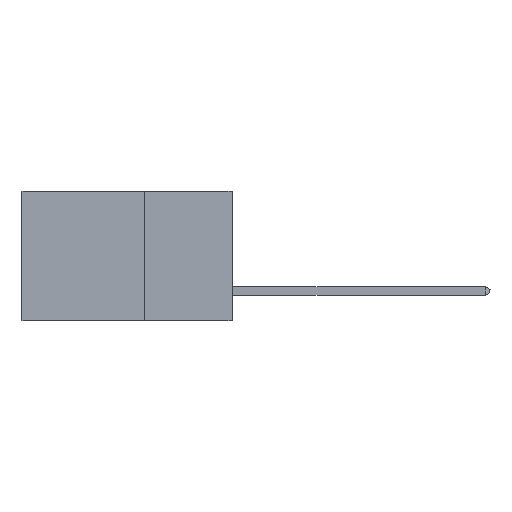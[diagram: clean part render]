
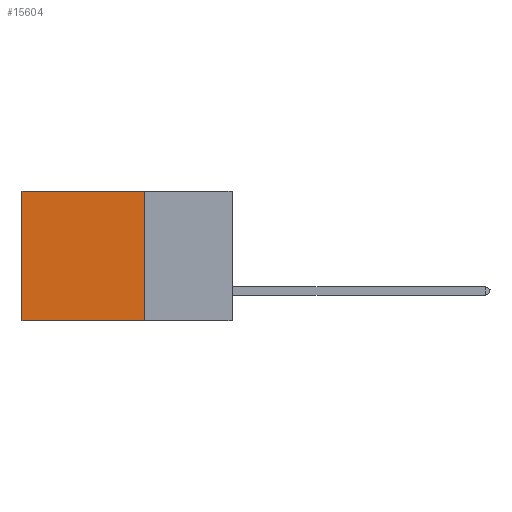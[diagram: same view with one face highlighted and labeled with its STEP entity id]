
A CAD part, left-side view. The second image highlights one B-rep face of the part: STEP entity #15604.
In plain terms, the highlighted planar face has unit normal (-1, 0, 0).
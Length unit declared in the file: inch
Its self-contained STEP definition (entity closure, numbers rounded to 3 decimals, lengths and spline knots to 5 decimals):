
#246 = CARTESIAN_POINT ( 'NONE',  ( 0.2875, 0.25, 0. ) ) ;
#857 = VECTOR ( 'NONE', #15147, 39.37008 ) ;
#1132 = EDGE_CURVE ( 'NONE', #14974, #2426, #4888, .T. ) ;
#1137 = LINE ( 'NONE', #3514, #15509 ) ;
#1570 = ORIENTED_EDGE ( 'NONE', *, *, #7758, .T. ) ;
#1942 = CARTESIAN_POINT ( 'NONE',  ( 0.2875, 0.25, -0.37 ) ) ;
#2011 = CARTESIAN_POINT ( 'NONE',  ( 0.2875, 0.6, 0. ) ) ;
#2426 = VERTEX_POINT ( 'NONE', #8627 ) ;
#2529 = AXIS2_PLACEMENT_3D ( 'NONE', #246, #14160, #15065 ) ;
#3514 = CARTESIAN_POINT ( 'NONE',  ( 0.2875, 0.25, 0. ) ) ;
#3666 = EDGE_LOOP ( 'NONE', ( #1570, #12010, #10888, #7827 ) ) ;
#4261 = CARTESIAN_POINT ( 'NONE',  ( 0.2875, 0.6, 0. ) ) ;
#4888 = LINE ( 'NONE', #7554, #12536 ) ;
#4927 = LINE ( 'NONE', #1942, #12577 ) ;
#5900 = LINE ( 'NONE', #4261, #857 ) ;
#7480 = CARTESIAN_POINT ( 'NONE',  ( 0.2875, 0.25, 0. ) ) ;
#7554 = CARTESIAN_POINT ( 'NONE',  ( 0.2875, 0.25, 0. ) ) ;
#7758 = EDGE_CURVE ( 'NONE', #17121, #17152, #5900, .T. ) ;
#7827 = ORIENTED_EDGE ( 'NONE', *, *, #10472, .T. ) ;
#8627 = CARTESIAN_POINT ( 'NONE',  ( 0.2875, 0.25, -0.37 ) ) ;
#10472 = EDGE_CURVE ( 'NONE', #14974, #17121, #1137, .T. ) ;
#10759 = DIRECTION ( 'NONE',  ( 0., 0., -1. ) ) ;
#10888 = ORIENTED_EDGE ( 'NONE', *, *, #1132, .F. ) ;
#12010 = ORIENTED_EDGE ( 'NONE', *, *, #17177, .F. ) ;
#12536 = VECTOR ( 'NONE', #10759, 39.37008 ) ;
#12577 = VECTOR ( 'NONE', #14186, 39.37008 ) ;
#12619 = DIRECTION ( 'NONE',  ( 0., 1., 0. ) ) ;
#14118 = CARTESIAN_POINT ( 'NONE',  ( 0.2875, 0.6, -0.37 ) ) ;
#14160 = DIRECTION ( 'NONE',  ( 1., 0., 0. ) ) ;
#14186 = DIRECTION ( 'NONE',  ( 0., 1., 0. ) ) ;
#14974 = VERTEX_POINT ( 'NONE', #7480 ) ;
#15065 = DIRECTION ( 'NONE',  ( 0., 0., -1. ) ) ;
#15147 = DIRECTION ( 'NONE',  ( 0., 0., -1. ) ) ;
#15509 = VECTOR ( 'NONE', #12619, 39.37008 ) ;
#15604 = ADVANCED_FACE ( 'NONE', ( #17719 ), #18601, .F. ) ;
#17121 = VERTEX_POINT ( 'NONE', #2011 ) ;
#17152 = VERTEX_POINT ( 'NONE', #14118 ) ;
#17177 = EDGE_CURVE ( 'NONE', #2426, #17152, #4927, .T. ) ;
#17719 = FACE_OUTER_BOUND ( 'NONE', #3666, .T. ) ;
#18601 = PLANE ( 'NONE',  #2529 ) ;
